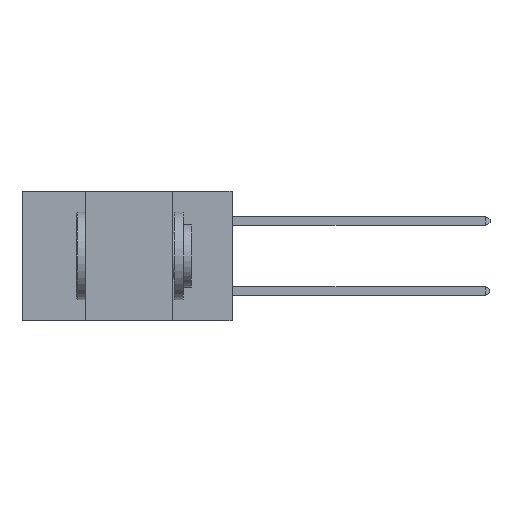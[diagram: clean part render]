
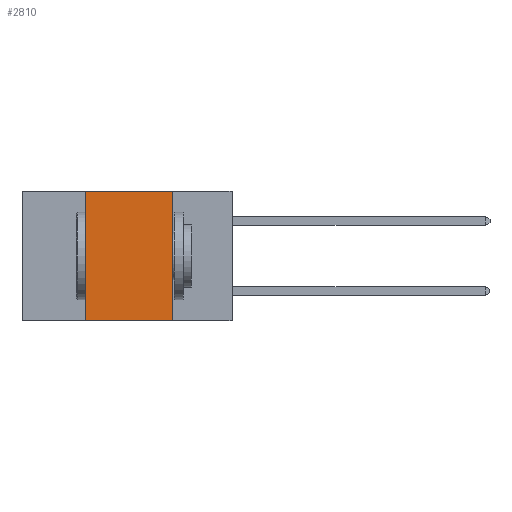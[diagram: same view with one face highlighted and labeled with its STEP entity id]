
A CAD part, left-side view. The second image highlights one B-rep face of the part: STEP entity #2810.
In plain terms, the highlighted planar face has unit normal (-1, 0, 0).
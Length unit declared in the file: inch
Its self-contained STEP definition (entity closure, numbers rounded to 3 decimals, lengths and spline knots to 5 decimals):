
#78 = VECTOR ( 'NONE', #3605, 39.37008 ) ;
#555 = DIRECTION ( 'NONE',  ( 0., 0., -1. ) ) ;
#821 = VECTOR ( 'NONE', #6643, 39.37008 ) ;
#1501 = ORIENTED_EDGE ( 'NONE', *, *, #5515, .T. ) ;
#1540 = ORIENTED_EDGE ( 'NONE', *, *, #9087, .F. ) ;
#1567 = VERTEX_POINT ( 'NONE', #3513 ) ;
#1643 = ORIENTED_EDGE ( 'NONE', *, *, #9519, .F. ) ;
#1765 = CARTESIAN_POINT ( 'NONE',  ( 0., 0.42, 0. ) ) ;
#1909 = DIRECTION ( 'NONE',  ( 0., 0., -1. ) ) ;
#1945 = DIRECTION ( 'NONE',  ( 1., 0., 0. ) ) ;
#2074 = PLANE ( 'NONE',  #7966 ) ;
#2188 = CARTESIAN_POINT ( 'NONE',  ( 0., 0.6, 0. ) ) ;
#2346 = EDGE_LOOP ( 'NONE', ( #6898, #1540, #1643, #1501 ) ) ;
#2471 = LINE ( 'NONE', #9933, #8180 ) ;
#2810 = ADVANCED_FACE ( 'NONE', ( #9102 ), #2074, .F. ) ;
#3174 = VERTEX_POINT ( 'NONE', #5421 ) ;
#3486 = LINE ( 'NONE', #10171, #821 ) ;
#3513 = CARTESIAN_POINT ( 'NONE',  ( 0., 0.17, 0. ) ) ;
#3605 = DIRECTION ( 'NONE',  ( 0., -1., 0. ) ) ;
#4463 = VERTEX_POINT ( 'NONE', #7655 ) ;
#5421 = CARTESIAN_POINT ( 'NONE',  ( 0., 0.17, -0.37 ) ) ;
#5515 = EDGE_CURVE ( 'NONE', #4463, #3174, #8187, .T. ) ;
#5569 = CARTESIAN_POINT ( 'NONE',  ( 0., 0.42, 0. ) ) ;
#5954 = CARTESIAN_POINT ( 'NONE',  ( 0., 0.6, -0.37 ) ) ;
#6292 = VECTOR ( 'NONE', #8465, 39.37008 ) ;
#6643 = DIRECTION ( 'NONE',  ( 0., -1., 0. ) ) ;
#6717 = EDGE_CURVE ( 'NONE', #1567, #3174, #2471, .T. ) ;
#6898 = ORIENTED_EDGE ( 'NONE', *, *, #6717, .F. ) ;
#7655 = CARTESIAN_POINT ( 'NONE',  ( 0., 0.42, -0.37 ) ) ;
#7966 = AXIS2_PLACEMENT_3D ( 'NONE', #2188, #1945, #1909 ) ;
#8180 = VECTOR ( 'NONE', #555, 39.37008 ) ;
#8187 = LINE ( 'NONE', #5954, #78 ) ;
#8196 = VERTEX_POINT ( 'NONE', #1765 ) ;
#8465 = DIRECTION ( 'NONE',  ( 0., 0., 1. ) ) ;
#9087 = EDGE_CURVE ( 'NONE', #8196, #1567, #3486, .T. ) ;
#9102 = FACE_OUTER_BOUND ( 'NONE', #2346, .T. ) ;
#9519 = EDGE_CURVE ( 'NONE', #4463, #8196, #9867, .T. ) ;
#9867 = LINE ( 'NONE', #5569, #6292 ) ;
#9933 = CARTESIAN_POINT ( 'NONE',  ( 0., 0.17, 0. ) ) ;
#10171 = CARTESIAN_POINT ( 'NONE',  ( 0., 0.6, 0. ) ) ;
